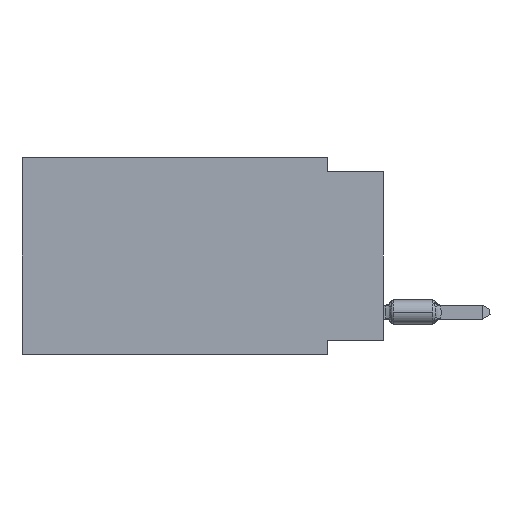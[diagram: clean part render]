
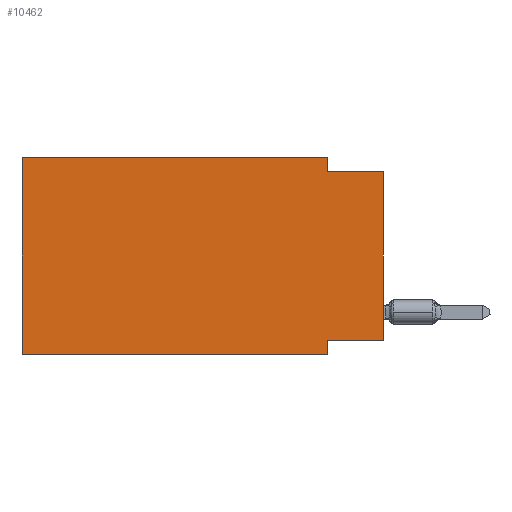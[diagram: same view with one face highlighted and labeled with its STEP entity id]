
A CAD part, left-side view. The second image highlights one B-rep face of the part: STEP entity #10462.
In plain terms, the highlighted planar face has unit normal (-1, 0, 0).
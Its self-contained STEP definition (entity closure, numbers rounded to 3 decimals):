
#1062 = VERTEX_POINT ( 'NONE', #32545 ) ;
#1764 = CARTESIAN_POINT ( 'NONE',  ( 0., 2.54, -0.635 ) ) ;
#2499 = CARTESIAN_POINT ( 'NONE',  ( 0., 0., -8.255 ) ) ;
#3076 = VERTEX_POINT ( 'NONE', #40571 ) ;
#3374 = CARTESIAN_POINT ( 'NONE',  ( 0., 16.383, -8.89 ) ) ;
#3999 = EDGE_CURVE ( 'NONE', #17124, #44890, #19325, .T. ) ;
#4489 = DIRECTION ( 'NONE',  ( 0., 0., 1. ) ) ;
#4923 = CARTESIAN_POINT ( 'NONE',  ( 0., 0., -0.635 ) ) ;
#5118 = LINE ( 'NONE', #32552, #55344 ) ;
#5299 = DIRECTION ( 'NONE',  ( 0., -1., 0. ) ) ;
#6002 = EDGE_CURVE ( 'NONE', #18303, #32103, #58852, .T. ) ;
#9680 = DIRECTION ( 'NONE',  ( 0., 0., -1. ) ) ;
#10462 = ADVANCED_FACE ( 'NONE', ( #54052 ), #34861, .F. ) ;
#13859 = VERTEX_POINT ( 'NONE', #1764 ) ;
#14143 = ORIENTED_EDGE ( 'NONE', *, *, #6002, .T. ) ;
#14772 = CARTESIAN_POINT ( 'NONE',  ( 0., 0., -0.635 ) ) ;
#15515 = DIRECTION ( 'NONE',  ( 0., -1., 0. ) ) ;
#17124 = VERTEX_POINT ( 'NONE', #2499 ) ;
#17630 = CARTESIAN_POINT ( 'NONE',  ( 0., 2.54, -8.89 ) ) ;
#18196 = EDGE_CURVE ( 'NONE', #13859, #44890, #23599, .T. ) ;
#18303 = VERTEX_POINT ( 'NONE', #47372 ) ;
#19225 = ORIENTED_EDGE ( 'NONE', *, *, #55504, .F. ) ;
#19325 = LINE ( 'NONE', #42799, #42679 ) ;
#20374 = VECTOR ( 'NONE', #39520, 1000. ) ;
#20632 = EDGE_CURVE ( 'NONE', #18303, #3076, #22495, .T. ) ;
#21756 = DIRECTION ( 'NONE',  ( 0., 0., -1. ) ) ;
#21831 = EDGE_CURVE ( 'NONE', #1062, #13859, #31635, .T. ) ;
#21928 = ORIENTED_EDGE ( 'NONE', *, *, #3999, .T. ) ;
#22495 = LINE ( 'NONE', #46269, #58936 ) ;
#22898 = ORIENTED_EDGE ( 'NONE', *, *, #53770, .F. ) ;
#23599 = LINE ( 'NONE', #14772, #46297 ) ;
#24652 = LINE ( 'NONE', #24935, #43707 ) ;
#24935 = CARTESIAN_POINT ( 'NONE',  ( 0., 16.383, 0. ) ) ;
#25184 = AXIS2_PLACEMENT_3D ( 'NONE', #26336, #35751, #21756 ) ;
#26336 = CARTESIAN_POINT ( 'NONE',  ( 0., 16.383, 0. ) ) ;
#27111 = VECTOR ( 'NONE', #50297, 1000. ) ;
#31343 = CARTESIAN_POINT ( 'NONE',  ( 0., 2.54, 0. ) ) ;
#31635 = LINE ( 'NONE', #31343, #44528 ) ;
#32103 = VERTEX_POINT ( 'NONE', #17630 ) ;
#32250 = EDGE_CURVE ( 'NONE', #56358, #32103, #5118, .T. ) ;
#32545 = CARTESIAN_POINT ( 'NONE',  ( 0., 2.54, 0. ) ) ;
#32552 = CARTESIAN_POINT ( 'NONE',  ( 0., 2.54, -8.89 ) ) ;
#33768 = LINE ( 'NONE', #52357, #20374 ) ;
#34736 = ORIENTED_EDGE ( 'NONE', *, *, #21831, .F. ) ;
#34861 = PLANE ( 'NONE',  #25184 ) ;
#35751 = DIRECTION ( 'NONE',  ( 1., 0., 0. ) ) ;
#36507 = DIRECTION ( 'NONE',  ( 0., 0., -1. ) ) ;
#36949 = ORIENTED_EDGE ( 'NONE', *, *, #20632, .F. ) ;
#39520 = DIRECTION ( 'NONE',  ( 0., 1., 0. ) ) ;
#40571 = CARTESIAN_POINT ( 'NONE',  ( 0., 16.383, 0. ) ) ;
#42270 = ORIENTED_EDGE ( 'NONE', *, *, #18196, .F. ) ;
#42679 = VECTOR ( 'NONE', #56815, 1000. ) ;
#42799 = CARTESIAN_POINT ( 'NONE',  ( 0., 0., 0. ) ) ;
#43339 = ORIENTED_EDGE ( 'NONE', *, *, #32250, .F. ) ;
#43707 = VECTOR ( 'NONE', #15515, 1000. ) ;
#44528 = VECTOR ( 'NONE', #36507, 1000. ) ;
#44890 = VERTEX_POINT ( 'NONE', #4923 ) ;
#46269 = CARTESIAN_POINT ( 'NONE',  ( 0., 16.383, 0. ) ) ;
#46297 = VECTOR ( 'NONE', #5299, 1000. ) ;
#47372 = CARTESIAN_POINT ( 'NONE',  ( 0., 16.383, -8.89 ) ) ;
#49044 = EDGE_LOOP ( 'NONE', ( #21928, #42270, #34736, #19225, #36949, #14143, #43339, #22898 ) ) ;
#50297 = DIRECTION ( 'NONE',  ( 0., -1., 0. ) ) ;
#52357 = CARTESIAN_POINT ( 'NONE',  ( 0., 0., -8.255 ) ) ;
#53770 = EDGE_CURVE ( 'NONE', #17124, #56358, #33768, .T. ) ;
#54052 = FACE_OUTER_BOUND ( 'NONE', #49044, .T. ) ;
#55344 = VECTOR ( 'NONE', #9680, 1000. ) ;
#55504 = EDGE_CURVE ( 'NONE', #3076, #1062, #24652, .T. ) ;
#56358 = VERTEX_POINT ( 'NONE', #56537 ) ;
#56537 = CARTESIAN_POINT ( 'NONE',  ( 0., 2.54, -8.255 ) ) ;
#56815 = DIRECTION ( 'NONE',  ( 0., 0., 1. ) ) ;
#58852 = LINE ( 'NONE', #3374, #27111 ) ;
#58936 = VECTOR ( 'NONE', #4489, 1000. ) ;
